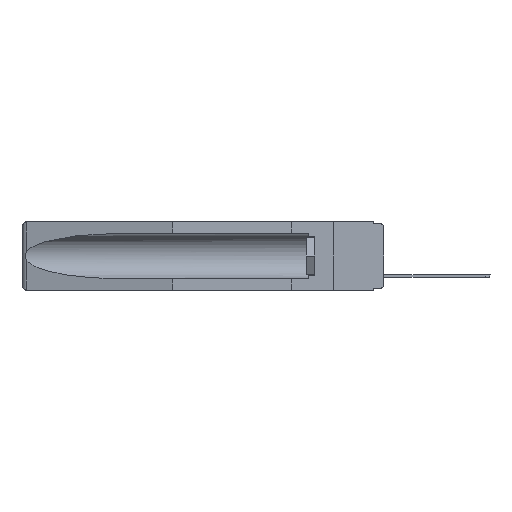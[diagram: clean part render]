
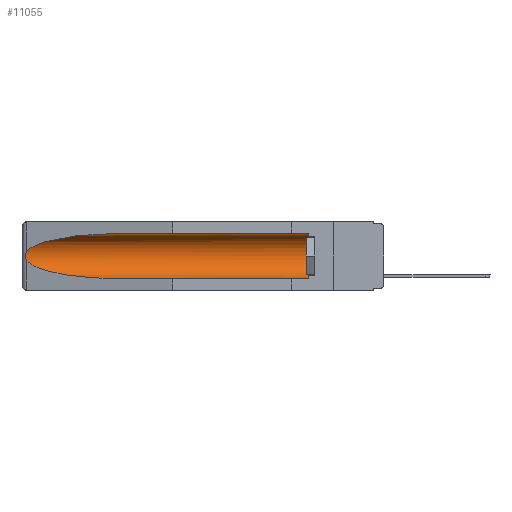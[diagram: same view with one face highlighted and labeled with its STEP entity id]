
A CAD part, left-side view. The second image highlights one B-rep face of the part: STEP entity #11055.
In plain terms, the highlighted cylindrical face has radius 2.857 mm (diameter 5.715 mm), a partial arc.
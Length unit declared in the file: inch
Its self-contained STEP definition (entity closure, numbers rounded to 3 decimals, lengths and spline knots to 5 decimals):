
#480 = CARTESIAN_POINT ( 'NONE',  ( 0.26537, 1.52718, -0.19328 ) ) ;
#1370 = CARTESIAN_POINT ( 'NONE',  ( 0.155, -0.30754, -0.059 ) ) ;
#1491 = CARTESIAN_POINT ( 'NONE',  ( 0.26537, 1.52718, -0.19328 ) ) ;
#2539 = VERTEX_POINT ( 'NONE', #13427 ) ;
#3508 = CARTESIAN_POINT ( 'NONE',  ( 0.26597, 1.52961, -0.15275 ) ) ;
#3648 = CARTESIAN_POINT ( 'NONE',  ( 0.155, 0.126, -0.1715 ) ) ;
#4289 = ORIENTED_EDGE ( 'NONE', *, *, #6833, .T. ) ;
#4383 = DIRECTION ( 'NONE',  ( 0., 1., 0. ) ) ;
#5647 = CARTESIAN_POINT ( 'NONE',  ( 0.26597, 1.5296, -0.19026 ) ) ;
#5737 = LINE ( 'NONE', #11883, #11208 ) ;
#6169 = CARTESIAN_POINT ( 'NONE',  ( 0.21114, 1.30732, -0.284 ) ) ;
#6515 = ORIENTED_EDGE ( 'NONE', *, *, #19051, .T. ) ;
#6833 = EDGE_CURVE ( 'NONE', #24713, #7899, #10262, .T. ) ;
#7243 = CARTESIAN_POINT ( 'NONE',  ( 0.155, 1.07973, -0.059 ) ) ;
#7899 = VERTEX_POINT ( 'NONE', #25038 ) ;
#8202 = CARTESIAN_POINT ( 'NONE',  ( 0.155, -0.30754, -0.1715 ) ) ;
#8538 = VERTEX_POINT ( 'NONE', #18035 ) ;
#9629 = CARTESIAN_POINT ( 'NONE',  ( 0.155, 1.07973, -0.059 ) ) ;
#9729 = AXIS2_PLACEMENT_3D ( 'NONE', #8202, #11973, #16149 ) ;
#10262 =( BOUNDED_CURVE ( )  B_SPLINE_CURVE ( 3, ( #9629, #17611, #23542, #19640 ),
 .UNSPECIFIED., .F., .F. ) 
 B_SPLINE_CURVE_WITH_KNOTS ( ( 4, 4 ),
 ( 4.71239, 6.08839 ),
 .UNSPECIFIED. ) 
 CURVE ( )  GEOMETRIC_REPRESENTATION_ITEM ( )  RATIONAL_B_SPLINE_CURVE ( ( 1., 0.848, 0.848, 1. ) ) 
 REPRESENTATION_ITEM ( '' )  );
#10324 = CARTESIAN_POINT ( 'NONE',  ( 0.25451, 1.48313, -0.24835 ) ) ;
#10907 = FACE_OUTER_BOUND ( 'NONE', #12720, .T. ) ;
#10993 = EDGE_CURVE ( 'NONE', #15303, #8538, #5737, .T. ) ;
#11055 = ADVANCED_FACE ( 'NONE', ( #10907 ), #12425, .F. ) ;
#11175 = CARTESIAN_POINT ( 'NONE',  ( 0.26655, 1.53094, -0.18657 ) ) ;
#11208 = VECTOR ( 'NONE', #4383, 39.37008 ) ;
#11261 = CARTESIAN_POINT ( 'NONE',  ( 0.26537, 1.52718, -0.14972 ) ) ;
#11722 = CIRCLE ( 'NONE', #15506, 0.1125 ) ;
#11883 = CARTESIAN_POINT ( 'NONE',  ( 0.155, -0.30754, -0.284 ) ) ;
#11973 = DIRECTION ( 'NONE',  ( 0., 1., 0. ) ) ;
#12425 = CYLINDRICAL_SURFACE ( 'NONE', #9729, 0.1125 ) ;
#12706 = VERTEX_POINT ( 'NONE', #18541 ) ;
#12720 = EDGE_LOOP ( 'NONE', ( #4289, #17306, #6515, #22966, #15564, #17292 ) ) ;
#13225 = CARTESIAN_POINT ( 'NONE',  ( 0.2675, 1.53308, -0.16763 ) ) ;
#13286 = DIRECTION ( 'NONE',  ( 0., 0., 1. ) ) ;
#13427 = CARTESIAN_POINT ( 'NONE',  ( 0.155, 0.126, -0.059 ) ) ;
#14105 = CARTESIAN_POINT ( 'NONE',  ( 0.155, 0.126, -0.284 ) ) ;
#14332 =( BOUNDED_CURVE ( )  B_SPLINE_CURVE ( 3, ( #480, #10324, #6169, #15791 ),
 .UNSPECIFIED., .F., .F. ) 
 B_SPLINE_CURVE_WITH_KNOTS ( ( 4, 4 ),
 ( 0.1948, 1.5708 ),
 .UNSPECIFIED. ) 
 CURVE ( )  GEOMETRIC_REPRESENTATION_ITEM ( )  RATIONAL_B_SPLINE_CURVE ( ( 1., 0.848, 0.848, 1. ) ) 
 REPRESENTATION_ITEM ( '' )  );
#15094 = CARTESIAN_POINT ( 'NONE',  ( 0.2673, 1.53269, -0.17917 ) ) ;
#15303 = VERTEX_POINT ( 'NONE', #14105 ) ;
#15506 = AXIS2_PLACEMENT_3D ( 'NONE', #3648, #23085, #13286 ) ;
#15564 = ORIENTED_EDGE ( 'NONE', *, *, #22661, .T. ) ;
#15570 = VECTOR ( 'NONE', #16791, 39.37008 ) ;
#15791 = CARTESIAN_POINT ( 'NONE',  ( 0.155, 1.07973, -0.284 ) ) ;
#16149 = DIRECTION ( 'NONE',  ( 0., 0., 1. ) ) ;
#16240 = B_SPLINE_CURVE_WITH_KNOTS ( 'NONE', 3,
 ( #11261, #3508, #25043, #21172, #13225, #17331, #15094, #11175, #5647, #1491 ),
 .UNSPECIFIED., .F., .F.,
 ( 4, 2, 2, 2, 4 ),
 ( 0., 0.00029, 0.00058, 0.00087, 0.00117 ),
 .UNSPECIFIED. ) ;
#16791 = DIRECTION ( 'NONE',  ( 0., 1., 0. ) ) ;
#17292 = ORIENTED_EDGE ( 'NONE', *, *, #20034, .T. ) ;
#17306 = ORIENTED_EDGE ( 'NONE', *, *, #22148, .T. ) ;
#17331 = CARTESIAN_POINT ( 'NONE',  ( 0.2675, 1.53308, -0.17534 ) ) ;
#17611 = CARTESIAN_POINT ( 'NONE',  ( 0.21114, 1.30732, -0.059 ) ) ;
#18035 = CARTESIAN_POINT ( 'NONE',  ( 0.155, 1.07973, -0.284 ) ) ;
#18541 = CARTESIAN_POINT ( 'NONE',  ( 0.26537, 1.52718, -0.19328 ) ) ;
#19051 = EDGE_CURVE ( 'NONE', #12706, #8538, #14332, .T. ) ;
#19640 = CARTESIAN_POINT ( 'NONE',  ( 0.26537, 1.52718, -0.14972 ) ) ;
#20034 = EDGE_CURVE ( 'NONE', #2539, #24713, #20763, .T. ) ;
#20763 = LINE ( 'NONE', #1370, #15570 ) ;
#21172 = CARTESIAN_POINT ( 'NONE',  ( 0.2673, 1.5327, -0.16383 ) ) ;
#22148 = EDGE_CURVE ( 'NONE', #7899, #12706, #16240, .T. ) ;
#22661 = EDGE_CURVE ( 'NONE', #15303, #2539, #11722, .T. ) ;
#22966 = ORIENTED_EDGE ( 'NONE', *, *, #10993, .F. ) ;
#23085 = DIRECTION ( 'NONE',  ( 0., -1., 0. ) ) ;
#23542 = CARTESIAN_POINT ( 'NONE',  ( 0.25451, 1.48313, -0.09465 ) ) ;
#24713 = VERTEX_POINT ( 'NONE', #7243 ) ;
#25038 = CARTESIAN_POINT ( 'NONE',  ( 0.26537, 1.52718, -0.14972 ) ) ;
#25043 = CARTESIAN_POINT ( 'NONE',  ( 0.26654, 1.53092, -0.15636 ) ) ;
